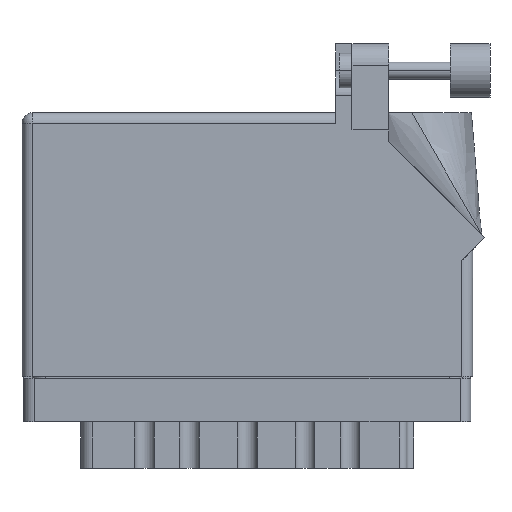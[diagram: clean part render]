
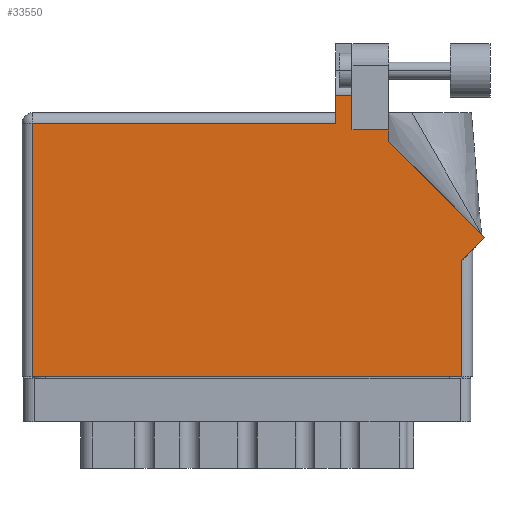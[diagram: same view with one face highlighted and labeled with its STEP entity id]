
A CAD part, front view. The second image highlights one B-rep face of the part: STEP entity #33550.
In plain terms, the highlighted face is planar.
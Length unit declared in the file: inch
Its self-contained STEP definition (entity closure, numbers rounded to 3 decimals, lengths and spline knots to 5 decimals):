
#323 = EDGE_CURVE ( 'NONE', #35536, #7975, #18034, .T. ) ;
#1099 = LINE ( 'NONE', #31567, #35707 ) ;
#1219 = VECTOR ( 'NONE', #13529, 39.37008 ) ;
#2902 = CARTESIAN_POINT ( 'NONE',  ( 2.55, 0., 0. ) ) ;
#4339 = ORIENTED_EDGE ( 'NONE', *, *, #43094, .T. ) ;
#4509 = CARTESIAN_POINT ( 'NONE',  ( 1.913, 1.43, 0. ) ) ;
#4894 = DIRECTION ( 'NONE',  ( 1., 0., 0. ) ) ;
#5220 = VECTOR ( 'NONE', #23242, 39.37008 ) ;
#5887 = ORIENTED_EDGE ( 'NONE', *, *, #27537, .T. ) ;
#5987 = LINE ( 'NONE', #43904, #1219 ) ;
#6133 = LINE ( 'NONE', #33615, #34189 ) ;
#6242 = ORIENTED_EDGE ( 'NONE', *, *, #11939, .T. ) ;
#7072 = LINE ( 'NONE', #31784, #43508 ) ;
#7837 = CARTESIAN_POINT ( 'NONE',  ( 1.913, 1.6315, 0. ) ) ;
#7975 = VERTEX_POINT ( 'NONE', #44859 ) ;
#8914 = LINE ( 'NONE', #36750, #48297 ) ;
#9610 = DIRECTION ( 'NONE',  ( 0., -1., 0. ) ) ;
#9849 = CARTESIAN_POINT ( 'NONE',  ( 1.819, 1.6315, 0. ) ) ;
#11592 = ORIENTED_EDGE ( 'NONE', *, *, #28701, .T. ) ;
#11939 = EDGE_CURVE ( 'NONE', #23054, #22925, #48216, .T. ) ;
#13439 = DIRECTION ( 'NONE',  ( -1., 0., 0. ) ) ;
#13529 = DIRECTION ( 'NONE',  ( 0., 1., 0. ) ) ;
#14346 = LINE ( 'NONE', #47808, #44184 ) ;
#15582 = PLANE ( 'NONE',  #24321 ) ;
#15903 = DIRECTION ( 'NONE',  ( 0., 0., -1. ) ) ;
#16165 = VECTOR ( 'NONE', #43562, 39.37008 ) ;
#17426 = ORIENTED_EDGE ( 'NONE', *, *, #35531, .T. ) ;
#18034 = LINE ( 'NONE', #37317, #21056 ) ;
#18105 = CARTESIAN_POINT ( 'NONE',  ( 2.126, 1.43, 0. ) ) ;
#18129 = VERTEX_POINT ( 'NONE', #2902 ) ;
#18644 = VECTOR ( 'NONE', #29501, 39.37008 ) ;
#19821 = LINE ( 'NONE', #44846, #18644 ) ;
#21056 = VECTOR ( 'NONE', #45169, 39.37008 ) ;
#22925 = VERTEX_POINT ( 'NONE', #18105 ) ;
#23054 = VERTEX_POINT ( 'NONE', #26603 ) ;
#23242 = DIRECTION ( 'NONE',  ( 0., 1., 0. ) ) ;
#23310 = VERTEX_POINT ( 'NONE', #24254 ) ;
#24046 = ORIENTED_EDGE ( 'NONE', *, *, #43467, .T. ) ;
#24254 = CARTESIAN_POINT ( 'NONE',  ( 0.062, 0., 0. ) ) ;
#24292 = VERTEX_POINT ( 'NONE', #37531 ) ;
#24297 = ORIENTED_EDGE ( 'NONE', *, *, #39229, .T. ) ;
#24321 = AXIS2_PLACEMENT_3D ( 'NONE', #38770, #15903, #41955 ) ;
#24634 = EDGE_CURVE ( 'NONE', #40052, #32562, #6133, .T. ) ;
#25519 = CARTESIAN_POINT ( 'NONE',  ( 1.819, 1.468, 0. ) ) ;
#26328 = LINE ( 'NONE', #32368, #16165 ) ;
#26603 = CARTESIAN_POINT ( 'NONE',  ( 2.126, 1.36442, 0. ) ) ;
#27178 = FACE_OUTER_BOUND ( 'NONE', #42360, .T. ) ;
#27537 = EDGE_CURVE ( 'NONE', #23310, #18129, #7072, .T. ) ;
#27814 = ORIENTED_EDGE ( 'NONE', *, *, #323, .T. ) ;
#28701 = EDGE_CURVE ( 'NONE', #32562, #35536, #30207, .T. ) ;
#29002 = VECTOR ( 'NONE', #9610, 39.37008 ) ;
#29159 = DIRECTION ( 'NONE',  ( -1., 0., 0. ) ) ;
#29501 = DIRECTION ( 'NONE',  ( 0., 1., 0. ) ) ;
#30207 = LINE ( 'NONE', #36440, #29002 ) ;
#30209 = VERTEX_POINT ( 'NONE', #4509 ) ;
#31567 = CARTESIAN_POINT ( 'NONE',  ( 2.612, 0.737, 0. ) ) ;
#31784 = CARTESIAN_POINT ( 'NONE',  ( 0., 0., 0. ) ) ;
#32343 = ORIENTED_EDGE ( 'NONE', *, *, #39311, .T. ) ;
#32368 = CARTESIAN_POINT ( 'NONE',  ( 2.68271, 0.80771, 0. ) ) ;
#32562 = VERTEX_POINT ( 'NONE', #9849 ) ;
#32739 = DIRECTION ( 'NONE',  ( 0., -1., 0. ) ) ;
#33550 = ADVANCED_FACE ( 'NONE', ( #27178 ), #15582, .F. ) ;
#33615 = CARTESIAN_POINT ( 'NONE',  ( 2.24377, 1.6315, 0. ) ) ;
#34189 = VECTOR ( 'NONE', #29159, 39.37008 ) ;
#34355 = CARTESIAN_POINT ( 'NONE',  ( 2.126, 1.36442, 0. ) ) ;
#35531 = EDGE_CURVE ( 'NONE', #30209, #40052, #19821, .T. ) ;
#35536 = VERTEX_POINT ( 'NONE', #25519 ) ;
#35707 = VECTOR ( 'NONE', #42576, 39.37008 ) ;
#36426 = CARTESIAN_POINT ( 'NONE',  ( 2.68271, 0.80771, 0. ) ) ;
#36440 = CARTESIAN_POINT ( 'NONE',  ( 1.819, 1.53, 0. ) ) ;
#36750 = CARTESIAN_POINT ( 'NONE',  ( 0.062, 0., 0. ) ) ;
#37317 = CARTESIAN_POINT ( 'NONE',  ( 0., 1.468, 0. ) ) ;
#37531 = CARTESIAN_POINT ( 'NONE',  ( 2.55, 0.675, 0. ) ) ;
#38770 = CARTESIAN_POINT ( 'NONE',  ( 0., 1.53, 0. ) ) ;
#39229 = EDGE_CURVE ( 'NONE', #47105, #23054, #26328, .T. ) ;
#39311 = EDGE_CURVE ( 'NONE', #18129, #24292, #5987, .T. ) ;
#40052 = VERTEX_POINT ( 'NONE', #7837 ) ;
#41032 = ORIENTED_EDGE ( 'NONE', *, *, #24634, .T. ) ;
#41698 = ORIENTED_EDGE ( 'NONE', *, *, #48624, .T. ) ;
#41955 = DIRECTION ( 'NONE',  ( -1., 0., 0. ) ) ;
#42360 = EDGE_LOOP ( 'NONE', ( #17426, #41032, #11592, #27814, #4339, #5887, #32343, #24046, #24297, #6242, #41698 ) ) ;
#42576 = DIRECTION ( 'NONE',  ( 0.707, 0.707, 0. ) ) ;
#43094 = EDGE_CURVE ( 'NONE', #7975, #23310, #8914, .T. ) ;
#43467 = EDGE_CURVE ( 'NONE', #24292, #47105, #1099, .T. ) ;
#43508 = VECTOR ( 'NONE', #4894, 39.37008 ) ;
#43562 = DIRECTION ( 'NONE',  ( -0.707, 0.707, 0. ) ) ;
#43904 = CARTESIAN_POINT ( 'NONE',  ( 2.55, 0.737, 0. ) ) ;
#44184 = VECTOR ( 'NONE', #13439, 39.37008 ) ;
#44846 = CARTESIAN_POINT ( 'NONE',  ( 1.913, 1.43, 0. ) ) ;
#44859 = CARTESIAN_POINT ( 'NONE',  ( 0.062, 1.468, 0. ) ) ;
#45169 = DIRECTION ( 'NONE',  ( -1., 0., 0. ) ) ;
#47105 = VERTEX_POINT ( 'NONE', #36426 ) ;
#47808 = CARTESIAN_POINT ( 'NONE',  ( 2.126, 1.43, 0. ) ) ;
#48216 = LINE ( 'NONE', #34355, #5220 ) ;
#48297 = VECTOR ( 'NONE', #32739, 39.37008 ) ;
#48624 = EDGE_CURVE ( 'NONE', #22925, #30209, #14346, .T. ) ;
